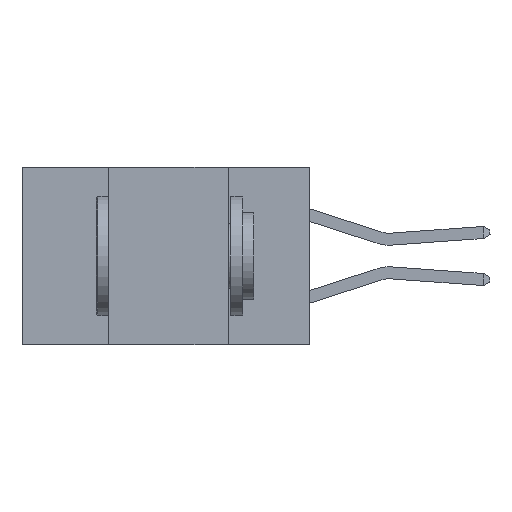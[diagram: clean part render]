
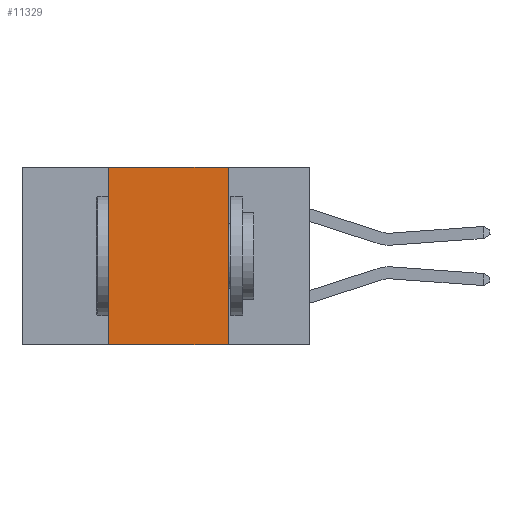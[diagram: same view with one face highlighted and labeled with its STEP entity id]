
A CAD part, left-side view. The second image highlights one B-rep face of the part: STEP entity #11329.
In plain terms, the highlighted planar face has unit normal (-1, 0, 0).
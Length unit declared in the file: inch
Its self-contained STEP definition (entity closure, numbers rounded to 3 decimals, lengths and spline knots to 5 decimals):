
#723 = AXIS2_PLACEMENT_3D ( 'NONE', #13840, #16071, #2918 ) ;
#1031 = LINE ( 'NONE', #5454, #6895 ) ;
#2918 = DIRECTION ( 'NONE',  ( 0., 0., -1. ) ) ;
#4225 = ORIENTED_EDGE ( 'NONE', *, *, #6298, .T. ) ;
#5175 = ORIENTED_EDGE ( 'NONE', *, *, #9637, .F. ) ;
#5454 = CARTESIAN_POINT ( 'NONE',  ( 0., 0.17, 0. ) ) ;
#5899 = LINE ( 'NONE', #12392, #16899 ) ;
#6298 = EDGE_CURVE ( 'NONE', #21212, #23055, #11668, .T. ) ;
#6895 = VECTOR ( 'NONE', #16290, 39.37008 ) ;
#9213 = EDGE_LOOP ( 'NONE', ( #21715, #28137, #5175, #4225 ) ) ;
#9637 = EDGE_CURVE ( 'NONE', #21212, #14804, #5899, .T. ) ;
#9981 = FACE_OUTER_BOUND ( 'NONE', #9213, .T. ) ;
#10724 = EDGE_CURVE ( 'NONE', #22521, #23055, #1031, .T. ) ;
#10969 = VECTOR ( 'NONE', #27007, 39.37008 ) ;
#11329 = ADVANCED_FACE ( 'NONE', ( #9981 ), #26879, .F. ) ;
#11668 = LINE ( 'NONE', #26979, #10969 ) ;
#11804 = DIRECTION ( 'NONE',  ( 0., -1., 0. ) ) ;
#12392 = CARTESIAN_POINT ( 'NONE',  ( 0., 0.42, 0. ) ) ;
#13840 = CARTESIAN_POINT ( 'NONE',  ( 0., 0.6, 0. ) ) ;
#14804 = VERTEX_POINT ( 'NONE', #16387 ) ;
#16071 = DIRECTION ( 'NONE',  ( 1., 0., 0. ) ) ;
#16290 = DIRECTION ( 'NONE',  ( 0., 0., -1. ) ) ;
#16387 = CARTESIAN_POINT ( 'NONE',  ( 0., 0.42, 0. ) ) ;
#16899 = VECTOR ( 'NONE', #21201, 39.37008 ) ;
#20013 = CARTESIAN_POINT ( 'NONE',  ( 0., 0.17, 0. ) ) ;
#20120 = EDGE_CURVE ( 'NONE', #14804, #22521, #26370, .T. ) ;
#20512 = CARTESIAN_POINT ( 'NONE',  ( 0., 0.6, 0. ) ) ;
#20631 = VECTOR ( 'NONE', #11804, 39.37008 ) ;
#20666 = CARTESIAN_POINT ( 'NONE',  ( 0., 0.17, -0.37 ) ) ;
#21201 = DIRECTION ( 'NONE',  ( 0., 0., 1. ) ) ;
#21212 = VERTEX_POINT ( 'NONE', #26215 ) ;
#21715 = ORIENTED_EDGE ( 'NONE', *, *, #10724, .F. ) ;
#22521 = VERTEX_POINT ( 'NONE', #20013 ) ;
#23055 = VERTEX_POINT ( 'NONE', #20666 ) ;
#26215 = CARTESIAN_POINT ( 'NONE',  ( 0., 0.42, -0.37 ) ) ;
#26370 = LINE ( 'NONE', #20512, #20631 ) ;
#26879 = PLANE ( 'NONE',  #723 ) ;
#26979 = CARTESIAN_POINT ( 'NONE',  ( 0., 0.6, -0.37 ) ) ;
#27007 = DIRECTION ( 'NONE',  ( 0., -1., 0. ) ) ;
#28137 = ORIENTED_EDGE ( 'NONE', *, *, #20120, .F. ) ;
